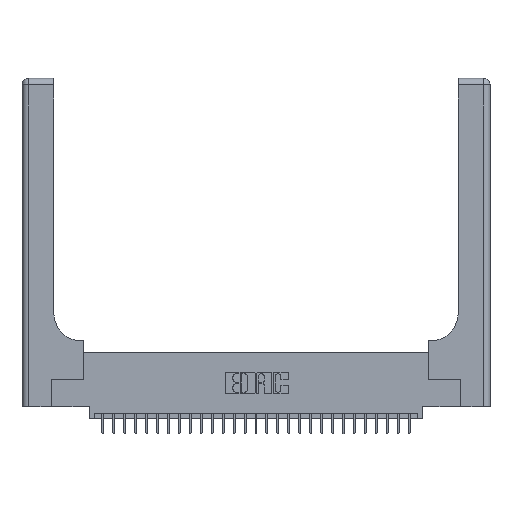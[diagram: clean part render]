
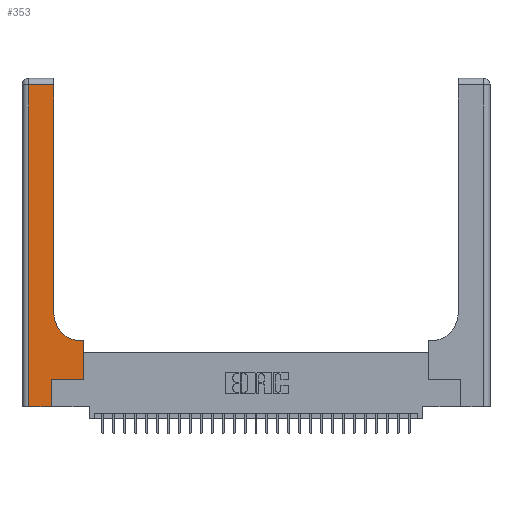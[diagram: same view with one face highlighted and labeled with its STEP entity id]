
A CAD part, top view. The second image highlights one B-rep face of the part: STEP entity #353.
In plain terms, the highlighted planar face has unit normal (0, 0, 1).
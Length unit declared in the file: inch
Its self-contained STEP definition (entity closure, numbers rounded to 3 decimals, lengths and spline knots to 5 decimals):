
#50 = LINE ( 'NONE', #16263, #11450 ) ;
#209 = CARTESIAN_POINT ( 'NONE',  ( 0.2915, 3., 0.37 ) ) ;
#353 = ADVANCED_FACE ( 'NONE', ( #4266 ), #15477, .F. ) ;
#613 = EDGE_CURVE ( 'NONE', #6801, #23736, #10028, .T. ) ;
#947 = AXIS2_PLACEMENT_3D ( 'NONE', #12597, #10606, #21955 ) ;
#1196 = VERTEX_POINT ( 'NONE', #9093 ) ;
#1482 = EDGE_LOOP ( 'NONE', ( #4846, #19969, #27758, #26249, #10885, #14628, #20549, #9480, #4384 ) ) ;
#2627 = CARTESIAN_POINT ( 'NONE',  ( 0.269, 0.25, 0.37 ) ) ;
#3267 = EDGE_CURVE ( 'NONE', #29536, #18310, #23164, .T. ) ;
#4127 = LINE ( 'NONE', #13389, #16148 ) ;
#4266 = FACE_OUTER_BOUND ( 'NONE', #1482, .T. ) ;
#4319 = EDGE_CURVE ( 'NONE', #18310, #15491, #20797, .T. ) ;
#4384 = ORIENTED_EDGE ( 'NONE', *, *, #3267, .T. ) ;
#4524 = CARTESIAN_POINT ( 'NONE',  ( 0.269, 0., 0.37 ) ) ;
#4846 = ORIENTED_EDGE ( 'NONE', *, *, #4319, .T. ) ;
#5276 = LINE ( 'NONE', #7422, #11261 ) ;
#6272 = DIRECTION ( 'NONE',  ( -1., 0., 0. ) ) ;
#6565 = EDGE_CURVE ( 'NONE', #7284, #29536, #5276, .T. ) ;
#6575 = DIRECTION ( 'NONE',  ( 0., 1., 0. ) ) ;
#6801 = VERTEX_POINT ( 'NONE', #14503 ) ;
#7108 = VERTEX_POINT ( 'NONE', #12511 ) ;
#7284 = VERTEX_POINT ( 'NONE', #13622 ) ;
#7312 = DIRECTION ( 'NONE',  ( 0., 1., 0. ) ) ;
#7422 = CARTESIAN_POINT ( 'NONE',  ( 0.2915, 0.6, 0.37 ) ) ;
#7742 = CARTESIAN_POINT ( 'NONE',  ( 0.2915, 2.94, 0.37 ) ) ;
#9093 = CARTESIAN_POINT ( 'NONE',  ( 0.5585, 0.25, 0.37 ) ) ;
#9467 = DIRECTION ( 'NONE',  ( 0., 1., 0. ) ) ;
#9480 = ORIENTED_EDGE ( 'NONE', *, *, #6565, .T. ) ;
#9514 = DIRECTION ( 'NONE',  ( 0., -1., 0. ) ) ;
#9664 = LINE ( 'NONE', #27796, #11327 ) ;
#9801 = CARTESIAN_POINT ( 'NONE',  ( 0.5415, 0.6, 0.37 ) ) ;
#10028 = LINE ( 'NONE', #19230, #15754 ) ;
#10312 = EDGE_CURVE ( 'NONE', #23736, #7108, #4127, .T. ) ;
#10606 = DIRECTION ( 'NONE',  ( 0., 0., -1. ) ) ;
#10835 = AXIS2_PLACEMENT_3D ( 'NONE', #24677, #18040, #6272 ) ;
#10885 = ORIENTED_EDGE ( 'NONE', *, *, #10312, .T. ) ;
#11261 = VECTOR ( 'NONE', #28389, 39.37008 ) ;
#11327 = VECTOR ( 'NONE', #9514, 39.37008 ) ;
#11450 = VECTOR ( 'NONE', #29881, 39.37008 ) ;
#11888 = DIRECTION ( 'NONE',  ( 1., 0., 0. ) ) ;
#12511 = CARTESIAN_POINT ( 'NONE',  ( 0.269, 0.25, 0.37 ) ) ;
#12597 = CARTESIAN_POINT ( 'NONE',  ( 0.5415, 0.85, 0.37 ) ) ;
#13164 = VECTOR ( 'NONE', #7312, 39.37008 ) ;
#13231 = EDGE_CURVE ( 'NONE', #15491, #15094, #50, .T. ) ;
#13389 = CARTESIAN_POINT ( 'NONE',  ( 0.269, 0., 0.37 ) ) ;
#13468 = EDGE_CURVE ( 'NONE', #7108, #1196, #23346, .T. ) ;
#13622 = CARTESIAN_POINT ( 'NONE',  ( 0.5585, 0.6, 0.37 ) ) ;
#14262 = LINE ( 'NONE', #16675, #13164 ) ;
#14503 = CARTESIAN_POINT ( 'NONE',  ( 0.06, 0., 0.37 ) ) ;
#14628 = ORIENTED_EDGE ( 'NONE', *, *, #13468, .T. ) ;
#15094 = VERTEX_POINT ( 'NONE', #16839 ) ;
#15477 = PLANE ( 'NONE',  #10835 ) ;
#15491 = VERTEX_POINT ( 'NONE', #7742 ) ;
#15754 = VECTOR ( 'NONE', #17139, 39.37008 ) ;
#16148 = VECTOR ( 'NONE', #6575, 39.37008 ) ;
#16263 = CARTESIAN_POINT ( 'NONE',  ( 0., 2.94, 0.37 ) ) ;
#16675 = CARTESIAN_POINT ( 'NONE',  ( 0.5585, 0.25, 0.37 ) ) ;
#16839 = CARTESIAN_POINT ( 'NONE',  ( 0.06, 2.94, 0.37 ) ) ;
#17139 = DIRECTION ( 'NONE',  ( 1., 0., 0. ) ) ;
#18040 = DIRECTION ( 'NONE',  ( 0., 0., -1. ) ) ;
#18310 = VERTEX_POINT ( 'NONE', #29195 ) ;
#19230 = CARTESIAN_POINT ( 'NONE',  ( 0., 0., 0.37 ) ) ;
#19969 = ORIENTED_EDGE ( 'NONE', *, *, #13231, .T. ) ;
#20549 = ORIENTED_EDGE ( 'NONE', *, *, #23340, .T. ) ;
#20797 = LINE ( 'NONE', #209, #24640 ) ;
#21955 = DIRECTION ( 'NONE',  ( 1., 0., 0. ) ) ;
#23164 = CIRCLE ( 'NONE', #947, 0.25 ) ;
#23340 = EDGE_CURVE ( 'NONE', #1196, #7284, #14262, .T. ) ;
#23346 = LINE ( 'NONE', #2627, #26406 ) ;
#23736 = VERTEX_POINT ( 'NONE', #4524 ) ;
#24640 = VECTOR ( 'NONE', #9467, 39.37008 ) ;
#24677 = CARTESIAN_POINT ( 'NONE',  ( 0., 3., 0.37 ) ) ;
#26249 = ORIENTED_EDGE ( 'NONE', *, *, #613, .T. ) ;
#26406 = VECTOR ( 'NONE', #11888, 39.37008 ) ;
#27758 = ORIENTED_EDGE ( 'NONE', *, *, #27929, .T. ) ;
#27796 = CARTESIAN_POINT ( 'NONE',  ( 0.06, 3., 0.37 ) ) ;
#27929 = EDGE_CURVE ( 'NONE', #15094, #6801, #9664, .T. ) ;
#28389 = DIRECTION ( 'NONE',  ( -1., 0., 0. ) ) ;
#29195 = CARTESIAN_POINT ( 'NONE',  ( 0.2915, 0.85, 0.37 ) ) ;
#29536 = VERTEX_POINT ( 'NONE', #9801 ) ;
#29881 = DIRECTION ( 'NONE',  ( -1., 0., 0. ) ) ;
